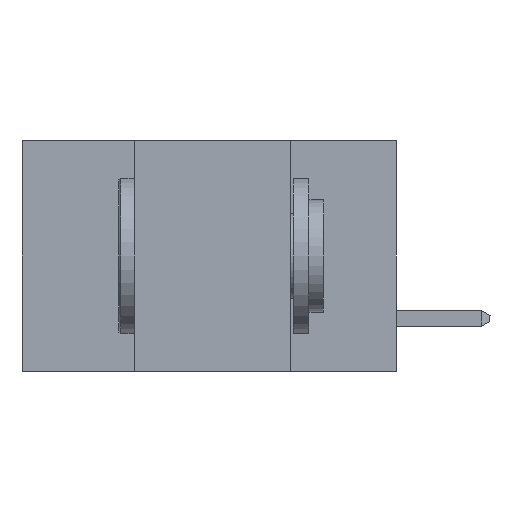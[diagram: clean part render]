
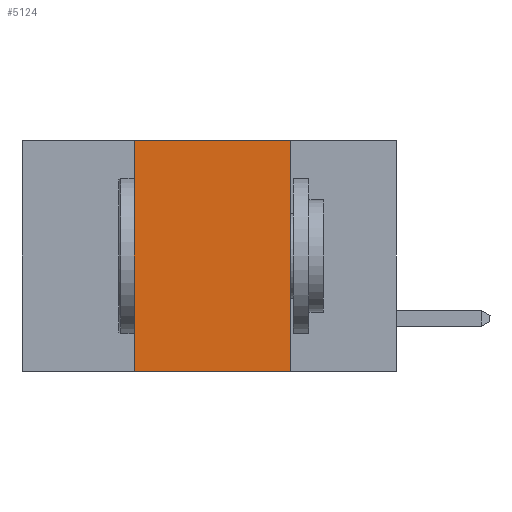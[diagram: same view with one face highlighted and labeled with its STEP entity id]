
A CAD part, left-side view. The second image highlights one B-rep face of the part: STEP entity #5124.
In plain terms, the highlighted planar face has unit normal (-1, 0, 0).
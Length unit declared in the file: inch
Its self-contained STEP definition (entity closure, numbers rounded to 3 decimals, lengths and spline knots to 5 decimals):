
#763 = LINE ( 'NONE', #11884, #1125 ) ;
#995 = EDGE_CURVE ( 'NONE', #1862, #11250, #11882, .T. ) ;
#1125 = VECTOR ( 'NONE', #7671, 39.37008 ) ;
#1127 = DIRECTION ( 'NONE',  ( 0., -1., 0. ) ) ;
#1862 = VERTEX_POINT ( 'NONE', #11713 ) ;
#2248 = AXIS2_PLACEMENT_3D ( 'NONE', #7831, #7960, #6847 ) ;
#2261 = EDGE_CURVE ( 'NONE', #10387, #1862, #763, .T. ) ;
#2926 = LINE ( 'NONE', #6131, #6883 ) ;
#3590 = VECTOR ( 'NONE', #9753, 39.37008 ) ;
#4619 = EDGE_LOOP ( 'NONE', ( #4992, #12588, #7073, #7600 ) ) ;
#4992 = ORIENTED_EDGE ( 'NONE', *, *, #11856, .F. ) ;
#5124 = ADVANCED_FACE ( 'NONE', ( #9363 ), #10873, .F. ) ;
#6131 = CARTESIAN_POINT ( 'NONE',  ( 0., 0.6, -0.37 ) ) ;
#6841 = LINE ( 'NONE', #10804, #3590 ) ;
#6847 = DIRECTION ( 'NONE',  ( 0., 0., -1. ) ) ;
#6883 = VECTOR ( 'NONE', #1127, 39.37008 ) ;
#7073 = ORIENTED_EDGE ( 'NONE', *, *, #2261, .F. ) ;
#7600 = ORIENTED_EDGE ( 'NONE', *, *, #8376, .T. ) ;
#7671 = DIRECTION ( 'NONE',  ( 0., 0., 1. ) ) ;
#7826 = VECTOR ( 'NONE', #9052, 39.37008 ) ;
#7831 = CARTESIAN_POINT ( 'NONE',  ( 0., 0.6, 0. ) ) ;
#7960 = DIRECTION ( 'NONE',  ( 1., 0., 0. ) ) ;
#8376 = EDGE_CURVE ( 'NONE', #10387, #10963, #2926, .T. ) ;
#9052 = DIRECTION ( 'NONE',  ( 0., -1., 0. ) ) ;
#9363 = FACE_OUTER_BOUND ( 'NONE', #4619, .T. ) ;
#9639 = CARTESIAN_POINT ( 'NONE',  ( 0., 0.17, 0. ) ) ;
#9735 = CARTESIAN_POINT ( 'NONE',  ( 0., 0.42, -0.37 ) ) ;
#9753 = DIRECTION ( 'NONE',  ( 0., 0., -1. ) ) ;
#10387 = VERTEX_POINT ( 'NONE', #9735 ) ;
#10804 = CARTESIAN_POINT ( 'NONE',  ( 0., 0.17, -0.37 ) ) ;
#10873 = PLANE ( 'NONE',  #2248 ) ;
#10963 = VERTEX_POINT ( 'NONE', #12973 ) ;
#10968 = CARTESIAN_POINT ( 'NONE',  ( 0., 0.6, 0. ) ) ;
#11250 = VERTEX_POINT ( 'NONE', #9639 ) ;
#11713 = CARTESIAN_POINT ( 'NONE',  ( 0., 0.42, 0. ) ) ;
#11856 = EDGE_CURVE ( 'NONE', #11250, #10963, #6841, .T. ) ;
#11882 = LINE ( 'NONE', #10968, #7826 ) ;
#11884 = CARTESIAN_POINT ( 'NONE',  ( 0., 0.42, -0.37 ) ) ;
#12588 = ORIENTED_EDGE ( 'NONE', *, *, #995, .F. ) ;
#12973 = CARTESIAN_POINT ( 'NONE',  ( 0., 0.17, -0.37 ) ) ;
